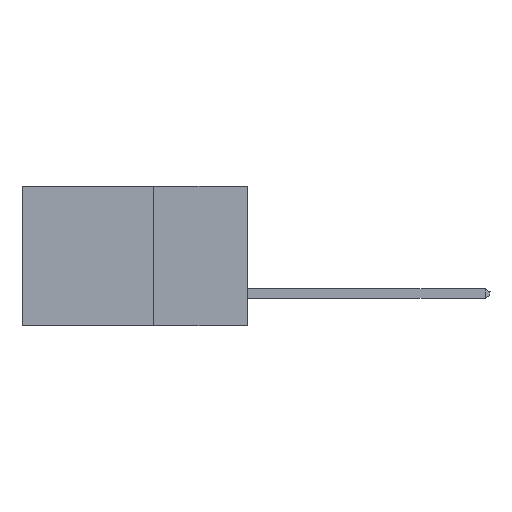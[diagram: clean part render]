
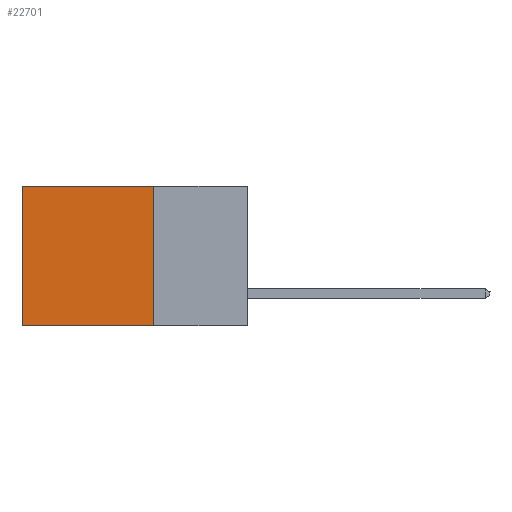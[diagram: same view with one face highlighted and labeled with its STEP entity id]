
A CAD part, left-side view. The second image highlights one B-rep face of the part: STEP entity #22701.
In plain terms, the highlighted planar face has unit normal (-1, 0, 0).
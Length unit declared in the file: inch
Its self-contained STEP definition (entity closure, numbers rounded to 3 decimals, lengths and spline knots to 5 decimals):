
#424 = AXIS2_PLACEMENT_3D ( 'NONE', #18082, #6672, #19895 ) ;
#1552 = CARTESIAN_POINT ( 'NONE',  ( 0.2615, 0.25, -0.37 ) ) ;
#1726 = CARTESIAN_POINT ( 'NONE',  ( 0.2615, 0.6, -0.37 ) ) ;
#1770 = DIRECTION ( 'NONE',  ( 0., 1., 0. ) ) ;
#2535 = EDGE_LOOP ( 'NONE', ( #6949, #16480, #13998, #17254 ) ) ;
#2558 = CARTESIAN_POINT ( 'NONE',  ( 0.2615, 0.25, -0.37 ) ) ;
#2899 = VERTEX_POINT ( 'NONE', #14230 ) ;
#3229 = FACE_OUTER_BOUND ( 'NONE', #2535, .T. ) ;
#4507 = CARTESIAN_POINT ( 'NONE',  ( 0.2615, 0.6, 0. ) ) ;
#4721 = PLANE ( 'NONE',  #424 ) ;
#6448 = EDGE_CURVE ( 'NONE', #16362, #10174, #12435, .T. ) ;
#6463 = DIRECTION ( 'NONE',  ( 0., 0., -1. ) ) ;
#6672 = DIRECTION ( 'NONE',  ( 1., 0., 0. ) ) ;
#6949 = ORIENTED_EDGE ( 'NONE', *, *, #6448, .T. ) ;
#7426 = DIRECTION ( 'NONE',  ( 0., 1., 0. ) ) ;
#7685 = EDGE_CURVE ( 'NONE', #2899, #10174, #10594, .T. ) ;
#8739 = EDGE_CURVE ( 'NONE', #18527, #16362, #10504, .T. ) ;
#10174 = VERTEX_POINT ( 'NONE', #1726 ) ;
#10504 = LINE ( 'NONE', #11218, #14415 ) ;
#10594 = LINE ( 'NONE', #1552, #15078 ) ;
#11218 = CARTESIAN_POINT ( 'NONE',  ( 0.2615, 0.25, 0. ) ) ;
#11767 = VECTOR ( 'NONE', #6463, 39.37008 ) ;
#12435 = LINE ( 'NONE', #14984, #22294 ) ;
#13998 = ORIENTED_EDGE ( 'NONE', *, *, #21328, .F. ) ;
#14230 = CARTESIAN_POINT ( 'NONE',  ( 0.2615, 0.25, -0.37 ) ) ;
#14415 = VECTOR ( 'NONE', #7426, 39.37008 ) ;
#14651 = DIRECTION ( 'NONE',  ( 0., 0., -1. ) ) ;
#14984 = CARTESIAN_POINT ( 'NONE',  ( 0.2615, 0.6, -0.37 ) ) ;
#15078 = VECTOR ( 'NONE', #1770, 39.37008 ) ;
#16362 = VERTEX_POINT ( 'NONE', #4507 ) ;
#16480 = ORIENTED_EDGE ( 'NONE', *, *, #7685, .F. ) ;
#16800 = LINE ( 'NONE', #2558, #11767 ) ;
#17254 = ORIENTED_EDGE ( 'NONE', *, *, #8739, .T. ) ;
#18082 = CARTESIAN_POINT ( 'NONE',  ( 0.2615, 0.25, -0.37 ) ) ;
#18527 = VERTEX_POINT ( 'NONE', #23938 ) ;
#19895 = DIRECTION ( 'NONE',  ( 0., 0., -1. ) ) ;
#21328 = EDGE_CURVE ( 'NONE', #18527, #2899, #16800, .T. ) ;
#22294 = VECTOR ( 'NONE', #14651, 39.37008 ) ;
#22701 = ADVANCED_FACE ( 'NONE', ( #3229 ), #4721, .F. ) ;
#23938 = CARTESIAN_POINT ( 'NONE',  ( 0.2615, 0.25, 0. ) ) ;
